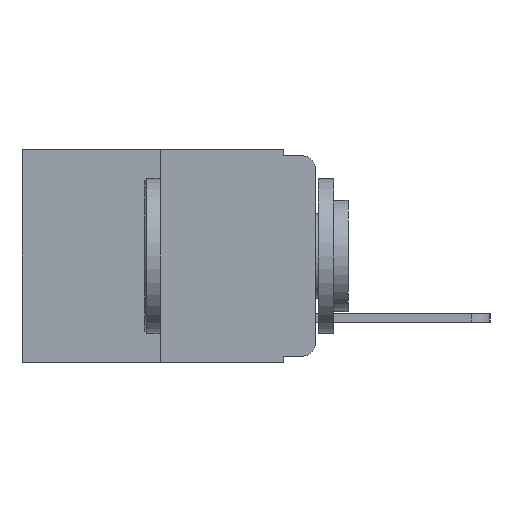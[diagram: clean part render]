
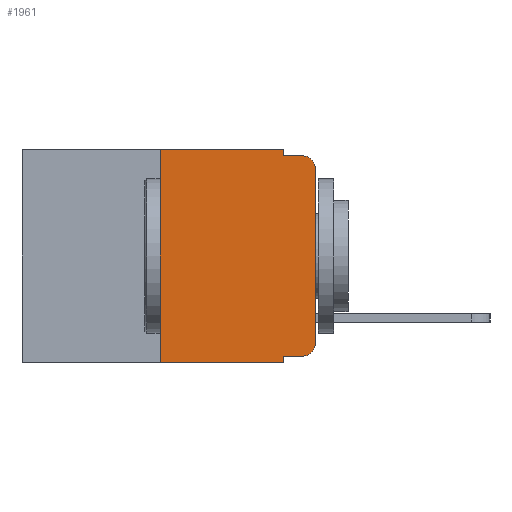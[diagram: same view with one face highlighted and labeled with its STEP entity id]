
A CAD part, left-side view. The second image highlights one B-rep face of the part: STEP entity #1961.
In plain terms, the highlighted planar face has unit normal (-1, 0, 0).
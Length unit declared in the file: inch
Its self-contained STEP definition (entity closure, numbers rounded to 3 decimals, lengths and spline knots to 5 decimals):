
#33 = CARTESIAN_POINT ( 'NONE',  ( 0., 0.051, -0.333 ) ) ;
#57 = DIRECTION ( 'NONE',  ( 0., 0., -1. ) ) ;
#225 = VERTEX_POINT ( 'NONE', #6939 ) ;
#456 = DIRECTION ( 'NONE',  ( 0., -1., 0. ) ) ;
#1221 = ORIENTED_EDGE ( 'NONE', *, *, #7664, .T. ) ;
#1339 = CARTESIAN_POINT ( 'NONE',  ( 0., 0., 0. ) ) ;
#1370 = DIRECTION ( 'NONE',  ( 0., 0., -1. ) ) ;
#1815 = LINE ( 'NONE', #9136, #8381 ) ;
#1872 = ORIENTED_EDGE ( 'NONE', *, *, #10059, .T. ) ;
#1961 = ADVANCED_FACE ( 'NONE', ( #7530 ), #9837, .F. ) ;
#2140 = CARTESIAN_POINT ( 'NONE',  ( 0., 0., -0.313 ) ) ;
#2147 = LINE ( 'NONE', #7112, #10723 ) ;
#2511 = VERTEX_POINT ( 'NONE', #8040 ) ;
#2575 = DIRECTION ( 'NONE',  ( 0., 0., 1. ) ) ;
#2685 = EDGE_CURVE ( 'NONE', #8534, #6127, #5240, .T. ) ;
#2844 = VECTOR ( 'NONE', #8007, 39.37008 ) ;
#2940 = VERTEX_POINT ( 'NONE', #7196 ) ;
#2952 = VECTOR ( 'NONE', #3556, 39.37008 ) ;
#3009 = CARTESIAN_POINT ( 'NONE',  ( 0., 0.051, 0. ) ) ;
#3189 = ORIENTED_EDGE ( 'NONE', *, *, #10844, .F. ) ;
#3556 = DIRECTION ( 'NONE',  ( 0., -1., 0. ) ) ;
#3699 = EDGE_CURVE ( 'NONE', #225, #6737, #7838, .T. ) ;
#3829 = CARTESIAN_POINT ( 'NONE',  ( 0., 0.051, -0.333 ) ) ;
#4019 = ORIENTED_EDGE ( 'NONE', *, *, #11122, .F. ) ;
#4323 = VERTEX_POINT ( 'NONE', #33 ) ;
#4392 = DIRECTION ( 'NONE',  ( 0., 0., -1. ) ) ;
#4446 = DIRECTION ( 'NONE',  ( 1., 0., 0. ) ) ;
#4559 = LINE ( 'NONE', #11040, #10743 ) ;
#4832 = EDGE_CURVE ( 'NONE', #9542, #225, #5734, .T. ) ;
#5000 = VECTOR ( 'NONE', #456, 39.37008 ) ;
#5071 = EDGE_CURVE ( 'NONE', #8345, #5647, #9523, .T. ) ;
#5240 = LINE ( 'NONE', #5889, #2844 ) ;
#5312 = VECTOR ( 'NONE', #57, 39.37008 ) ;
#5467 = VECTOR ( 'NONE', #2575, 39.37008 ) ;
#5490 = AXIS2_PLACEMENT_3D ( 'NONE', #5624, #5561, #1370 ) ;
#5561 = DIRECTION ( 'NONE',  ( -1., 0., 0. ) ) ;
#5624 = CARTESIAN_POINT ( 'NONE',  ( 0., 0.02, -0.313 ) ) ;
#5647 = VERTEX_POINT ( 'NONE', #10830 ) ;
#5734 = LINE ( 'NONE', #1339, #5467 ) ;
#5889 = CARTESIAN_POINT ( 'NONE',  ( 0., 0.25, 0. ) ) ;
#6127 = VERTEX_POINT ( 'NONE', #9985 ) ;
#6203 = CARTESIAN_POINT ( 'NONE',  ( 0., 0.25, -0.343 ) ) ;
#6342 = DIRECTION ( 'NONE',  ( 0., 0., -1. ) ) ;
#6721 = ORIENTED_EDGE ( 'NONE', *, *, #4832, .T. ) ;
#6737 = VERTEX_POINT ( 'NONE', #9634 ) ;
#6791 = AXIS2_PLACEMENT_3D ( 'NONE', #10995, #4446, #4392 ) ;
#6939 = CARTESIAN_POINT ( 'NONE',  ( 0., 0., -0.03 ) ) ;
#6948 = EDGE_CURVE ( 'NONE', #2511, #9542, #9968, .T. ) ;
#7056 = DIRECTION ( 'NONE',  ( 0., 0., -1. ) ) ;
#7074 = DIRECTION ( 'NONE',  ( -1., 0., 0. ) ) ;
#7081 = EDGE_LOOP ( 'NONE', ( #6721, #10891, #9071, #11111, #3189, #7697, #1221, #4019, #1872, #10774 ) ) ;
#7112 = CARTESIAN_POINT ( 'NONE',  ( 0., 0.051, -0.01 ) ) ;
#7195 = LINE ( 'NONE', #9966, #5000 ) ;
#7196 = CARTESIAN_POINT ( 'NONE',  ( 0., 0.051, -0.343 ) ) ;
#7320 = DIRECTION ( 'NONE',  ( 0., -1., 0. ) ) ;
#7530 = FACE_OUTER_BOUND ( 'NONE', #7081, .T. ) ;
#7664 = EDGE_CURVE ( 'NONE', #8534, #2940, #1815, .T. ) ;
#7697 = ORIENTED_EDGE ( 'NONE', *, *, #2685, .F. ) ;
#7758 = CARTESIAN_POINT ( 'NONE',  ( 0., 0.051, 0. ) ) ;
#7778 = AXIS2_PLACEMENT_3D ( 'NONE', #9315, #7074, #7056 ) ;
#7838 = CIRCLE ( 'NONE', #7778, 0.02 ) ;
#8007 = DIRECTION ( 'NONE',  ( 0., 0., 1. ) ) ;
#8040 = CARTESIAN_POINT ( 'NONE',  ( 0., 0.02, -0.333 ) ) ;
#8092 = EDGE_CURVE ( 'NONE', #5647, #6737, #2147, .T. ) ;
#8345 = VERTEX_POINT ( 'NONE', #7758 ) ;
#8381 = VECTOR ( 'NONE', #9457, 39.37008 ) ;
#8534 = VERTEX_POINT ( 'NONE', #6203 ) ;
#9071 = ORIENTED_EDGE ( 'NONE', *, *, #8092, .F. ) ;
#9136 = CARTESIAN_POINT ( 'NONE',  ( 0., 0.473, -0.343 ) ) ;
#9315 = CARTESIAN_POINT ( 'NONE',  ( 0., 0.02, -0.03 ) ) ;
#9457 = DIRECTION ( 'NONE',  ( 0., -1., 0. ) ) ;
#9523 = LINE ( 'NONE', #3009, #5312 ) ;
#9542 = VERTEX_POINT ( 'NONE', #2140 ) ;
#9551 = LINE ( 'NONE', #3829, #2952 ) ;
#9634 = CARTESIAN_POINT ( 'NONE',  ( 0., 0.02, -0.01 ) ) ;
#9837 = PLANE ( 'NONE',  #6791 ) ;
#9966 = CARTESIAN_POINT ( 'NONE',  ( 0., 0.473, 0. ) ) ;
#9968 = CIRCLE ( 'NONE', #5490, 0.02 ) ;
#9985 = CARTESIAN_POINT ( 'NONE',  ( 0., 0.25, 0. ) ) ;
#10059 = EDGE_CURVE ( 'NONE', #4323, #2511, #9551, .T. ) ;
#10723 = VECTOR ( 'NONE', #7320, 39.37008 ) ;
#10743 = VECTOR ( 'NONE', #6342, 39.37008 ) ;
#10774 = ORIENTED_EDGE ( 'NONE', *, *, #6948, .T. ) ;
#10830 = CARTESIAN_POINT ( 'NONE',  ( 0., 0.051, -0.01 ) ) ;
#10844 = EDGE_CURVE ( 'NONE', #6127, #8345, #7195, .T. ) ;
#10891 = ORIENTED_EDGE ( 'NONE', *, *, #3699, .T. ) ;
#10995 = CARTESIAN_POINT ( 'NONE',  ( 0., 0.473, 0. ) ) ;
#11040 = CARTESIAN_POINT ( 'NONE',  ( 0., 0.051, 0. ) ) ;
#11111 = ORIENTED_EDGE ( 'NONE', *, *, #5071, .F. ) ;
#11122 = EDGE_CURVE ( 'NONE', #4323, #2940, #4559, .T. ) ;
